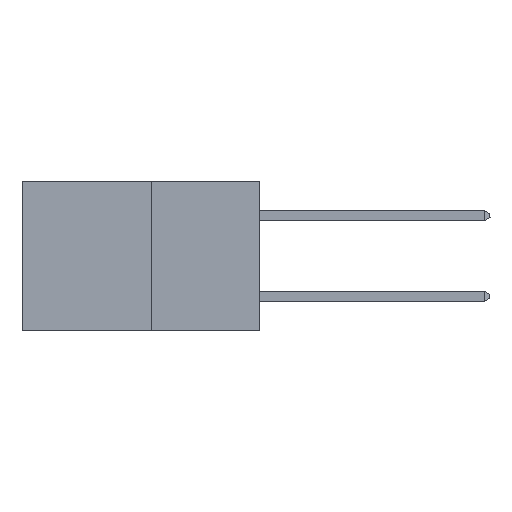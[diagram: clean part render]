
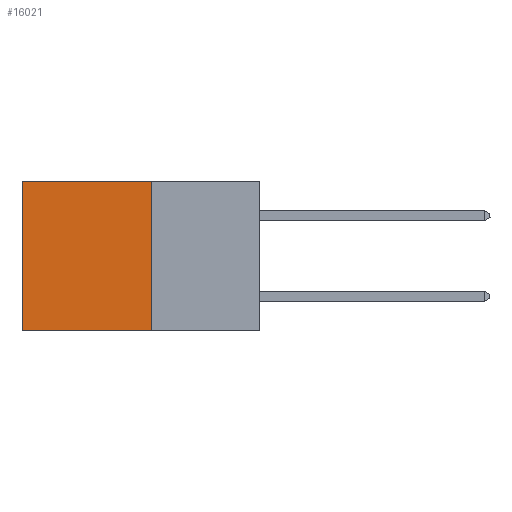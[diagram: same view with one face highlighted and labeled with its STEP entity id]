
A CAD part, left-side view. The second image highlights one B-rep face of the part: STEP entity #16021.
In plain terms, the highlighted planar face has unit normal (-1, 0, 0).
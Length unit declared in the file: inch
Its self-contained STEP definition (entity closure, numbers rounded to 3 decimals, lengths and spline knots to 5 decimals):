
#9 = LINE ( 'NONE', #15162, #4086 ) ;
#1419 = DIRECTION ( 'NONE',  ( 1., 0., 0. ) ) ;
#1958 = DIRECTION ( 'NONE',  ( 0., 0., -1. ) ) ;
#2097 = CARTESIAN_POINT ( 'NONE',  ( 0.277, 0.27, -0.37 ) ) ;
#2121 = EDGE_LOOP ( 'NONE', ( #11029, #4768, #15451, #6416 ) ) ;
#2349 = VECTOR ( 'NONE', #3971, 39.37008 ) ;
#2799 = CARTESIAN_POINT ( 'NONE',  ( 0.277, 0.59, 0. ) ) ;
#2931 = EDGE_CURVE ( 'NONE', #10591, #7715, #5461, .T. ) ;
#2989 = VERTEX_POINT ( 'NONE', #4713 ) ;
#3971 = DIRECTION ( 'NONE',  ( 0., 1., 0. ) ) ;
#4046 = CARTESIAN_POINT ( 'NONE',  ( 0.277, 0.27, 0. ) ) ;
#4056 = CARTESIAN_POINT ( 'NONE',  ( 0.277, 0.27, -0.37 ) ) ;
#4086 = VECTOR ( 'NONE', #1958, 39.37008 ) ;
#4456 = DIRECTION ( 'NONE',  ( 0., 1., 0. ) ) ;
#4713 = CARTESIAN_POINT ( 'NONE',  ( 0.277, 0.59, -0.37 ) ) ;
#4768 = ORIENTED_EDGE ( 'NONE', *, *, #12131, .F. ) ;
#5153 = CARTESIAN_POINT ( 'NONE',  ( 0.277, 0.27, 0. ) ) ;
#5461 = LINE ( 'NONE', #4046, #2349 ) ;
#6416 = ORIENTED_EDGE ( 'NONE', *, *, #2931, .T. ) ;
#7215 = FACE_OUTER_BOUND ( 'NONE', #2121, .T. ) ;
#7715 = VERTEX_POINT ( 'NONE', #2799 ) ;
#9085 = LINE ( 'NONE', #2097, #12643 ) ;
#9307 = PLANE ( 'NONE',  #10527 ) ;
#9730 = CARTESIAN_POINT ( 'NONE',  ( 0.277, 0.27, -0.37 ) ) ;
#9928 = DIRECTION ( 'NONE',  ( 0., 0., -1. ) ) ;
#10527 = AXIS2_PLACEMENT_3D ( 'NONE', #4056, #1419, #10659 ) ;
#10591 = VERTEX_POINT ( 'NONE', #5153 ) ;
#10659 = DIRECTION ( 'NONE',  ( 0., 0., -1. ) ) ;
#11029 = ORIENTED_EDGE ( 'NONE', *, *, #12642, .T. ) ;
#11635 = CARTESIAN_POINT ( 'NONE',  ( 0.277, 0.27, -0.37 ) ) ;
#11789 = VERTEX_POINT ( 'NONE', #11635 ) ;
#12131 = EDGE_CURVE ( 'NONE', #11789, #2989, #17064, .T. ) ;
#12642 = EDGE_CURVE ( 'NONE', #7715, #2989, #9, .T. ) ;
#12643 = VECTOR ( 'NONE', #9928, 39.37008 ) ;
#13605 = VECTOR ( 'NONE', #4456, 39.37008 ) ;
#15162 = CARTESIAN_POINT ( 'NONE',  ( 0.277, 0.59, -0.37 ) ) ;
#15451 = ORIENTED_EDGE ( 'NONE', *, *, #15696, .F. ) ;
#15696 = EDGE_CURVE ( 'NONE', #10591, #11789, #9085, .T. ) ;
#16021 = ADVANCED_FACE ( 'NONE', ( #7215 ), #9307, .F. ) ;
#17064 = LINE ( 'NONE', #9730, #13605 ) ;
